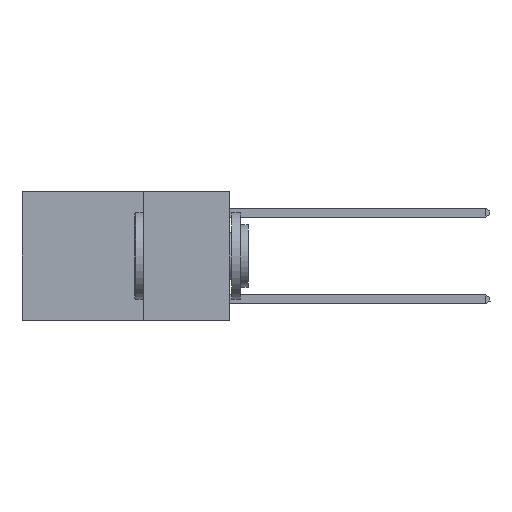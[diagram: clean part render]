
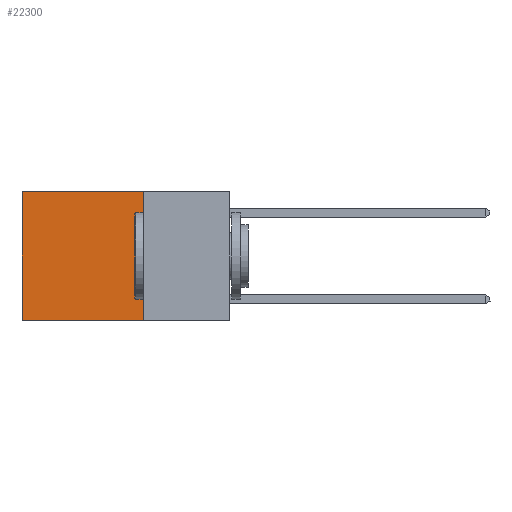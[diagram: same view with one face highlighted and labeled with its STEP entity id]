
A CAD part, left-side view. The second image highlights one B-rep face of the part: STEP entity #22300.
In plain terms, the highlighted planar face has unit normal (-1, 0, 0).
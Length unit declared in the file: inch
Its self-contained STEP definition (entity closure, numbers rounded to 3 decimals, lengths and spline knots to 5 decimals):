
#607 = AXIS2_PLACEMENT_3D ( 'NONE', #9810, #29042, #14682 ) ;
#983 = VECTOR ( 'NONE', #6616, 39.37008 ) ;
#1630 = CARTESIAN_POINT ( 'NONE',  ( 0.2625, 0.6, 0. ) ) ;
#1859 = CARTESIAN_POINT ( 'NONE',  ( 0.2625, 0.25, -0.37 ) ) ;
#3190 = EDGE_CURVE ( 'NONE', #26458, #8576, #4401, .T. ) ;
#3482 = VECTOR ( 'NONE', #11640, 39.37008 ) ;
#3485 = CARTESIAN_POINT ( 'NONE',  ( 0.2625, 0.6, 0. ) ) ;
#4401 = LINE ( 'NONE', #23989, #28542 ) ;
#6616 = DIRECTION ( 'NONE',  ( 0., 0., -1. ) ) ;
#7857 = EDGE_LOOP ( 'NONE', ( #9874, #16842, #26784, #9280 ) ) ;
#8033 = EDGE_CURVE ( 'NONE', #8576, #24745, #26675, .T. ) ;
#8576 = VERTEX_POINT ( 'NONE', #3485 ) ;
#9280 = ORIENTED_EDGE ( 'NONE', *, *, #3190, .T. ) ;
#9304 = DIRECTION ( 'NONE',  ( 0., 0., -1. ) ) ;
#9810 = CARTESIAN_POINT ( 'NONE',  ( 0.2625, 0.25, 0. ) ) ;
#9874 = ORIENTED_EDGE ( 'NONE', *, *, #8033, .T. ) ;
#9942 = FACE_OUTER_BOUND ( 'NONE', #7857, .T. ) ;
#9960 = LINE ( 'NONE', #1859, #3482 ) ;
#10515 = EDGE_CURVE ( 'NONE', #16600, #24745, #9960, .T. ) ;
#10555 = EDGE_CURVE ( 'NONE', #26458, #16600, #15629, .T. ) ;
#11640 = DIRECTION ( 'NONE',  ( 0., 1., 0. ) ) ;
#12560 = CARTESIAN_POINT ( 'NONE',  ( 0.2625, 0.6, -0.37 ) ) ;
#14682 = DIRECTION ( 'NONE',  ( 0., 0., -1. ) ) ;
#15504 = CARTESIAN_POINT ( 'NONE',  ( 0.2625, 0.25, -0.37 ) ) ;
#15629 = LINE ( 'NONE', #30916, #17154 ) ;
#16600 = VERTEX_POINT ( 'NONE', #15504 ) ;
#16842 = ORIENTED_EDGE ( 'NONE', *, *, #10515, .F. ) ;
#17154 = VECTOR ( 'NONE', #9304, 39.37008 ) ;
#19292 = DIRECTION ( 'NONE',  ( 0., 1., 0. ) ) ;
#22300 = ADVANCED_FACE ( 'NONE', ( #9942 ), #26629, .F. ) ;
#23989 = CARTESIAN_POINT ( 'NONE',  ( 0.2625, 0.25, 0. ) ) ;
#24745 = VERTEX_POINT ( 'NONE', #12560 ) ;
#26458 = VERTEX_POINT ( 'NONE', #30828 ) ;
#26629 = PLANE ( 'NONE',  #607 ) ;
#26675 = LINE ( 'NONE', #1630, #983 ) ;
#26784 = ORIENTED_EDGE ( 'NONE', *, *, #10555, .F. ) ;
#28542 = VECTOR ( 'NONE', #19292, 39.37008 ) ;
#29042 = DIRECTION ( 'NONE',  ( 1., 0., 0. ) ) ;
#30828 = CARTESIAN_POINT ( 'NONE',  ( 0.2625, 0.25, 0. ) ) ;
#30916 = CARTESIAN_POINT ( 'NONE',  ( 0.2625, 0.25, 0. ) ) ;
